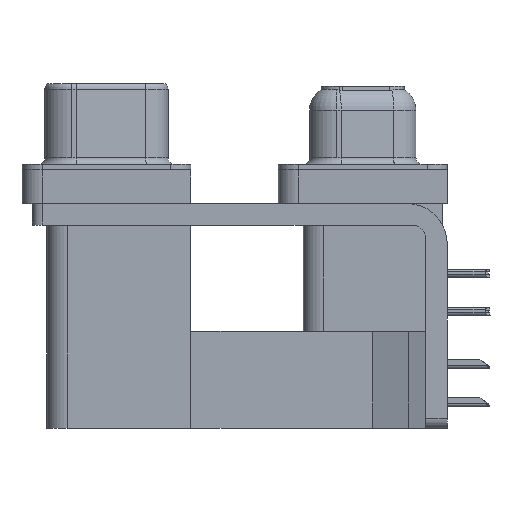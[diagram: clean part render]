
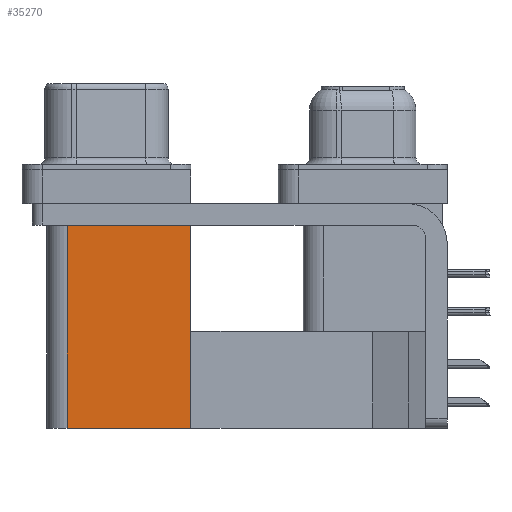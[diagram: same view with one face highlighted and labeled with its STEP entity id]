
A CAD part, left-side view. The second image highlights one B-rep face of the part: STEP entity #35270.
In plain terms, the highlighted planar face has unit normal (-1, 0, 0).
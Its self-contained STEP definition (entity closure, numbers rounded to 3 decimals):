
#54 = ORIENTED_EDGE ( 'NONE', *, *, #5511, .F. ) ;
#746 = FACE_OUTER_BOUND ( 'NONE', #6804, .T. ) ;
#1076 = VECTOR ( 'NONE', #1317, 1000. ) ;
#1317 = DIRECTION ( 'NONE',  ( 0., 1., 0. ) ) ;
#1485 = DIRECTION ( 'NONE',  ( 1., 0., 0. ) ) ;
#1719 = DIRECTION ( 'NONE',  ( 0., 0., 1. ) ) ;
#4281 = VERTEX_POINT ( 'NONE', #9733 ) ;
#5478 = LINE ( 'NONE', #19414, #6993 ) ;
#5511 = EDGE_CURVE ( 'NONE', #35885, #22457, #18679, .T. ) ;
#6804 = EDGE_LOOP ( 'NONE', ( #35954, #54, #20060, #24211 ) ) ;
#6993 = VECTOR ( 'NONE', #16777, 1000. ) ;
#9494 = EDGE_CURVE ( 'NONE', #33871, #35885, #5478, .T. ) ;
#9733 = CARTESIAN_POINT ( 'NONE',  ( 3.79, 12.775, -2.5 ) ) ;
#11912 = LINE ( 'NONE', #17920, #20626 ) ;
#12416 = CARTESIAN_POINT ( 'NONE',  ( 3.79, 21.975, -2.5 ) ) ;
#12964 = DIRECTION ( 'NONE',  ( 0., 0., -1. ) ) ;
#16777 = DIRECTION ( 'NONE',  ( 0., 1., 0. ) ) ;
#17920 = CARTESIAN_POINT ( 'NONE',  ( 3.79, 12.775, -19.2 ) ) ;
#18240 = EDGE_CURVE ( 'NONE', #33871, #4281, #11912, .T. ) ;
#18679 = LINE ( 'NONE', #33002, #27005 ) ;
#19414 = CARTESIAN_POINT ( 'NONE',  ( 3.79, 12.775, -19.2 ) ) ;
#20060 = ORIENTED_EDGE ( 'NONE', *, *, #9494, .F. ) ;
#20626 = VECTOR ( 'NONE', #32243, 1000. ) ;
#22457 = VERTEX_POINT ( 'NONE', #12416 ) ;
#24211 = ORIENTED_EDGE ( 'NONE', *, *, #18240, .T. ) ;
#27005 = VECTOR ( 'NONE', #1719, 1000. ) ;
#27107 = CARTESIAN_POINT ( 'NONE',  ( 3.79, 12.775, -19.2 ) ) ;
#28250 = AXIS2_PLACEMENT_3D ( 'NONE', #27107, #1485, #12964 ) ;
#28579 = CARTESIAN_POINT ( 'NONE',  ( 3.79, 12.775, -19.2 ) ) ;
#31033 = EDGE_CURVE ( 'NONE', #4281, #22457, #32777, .T. ) ;
#32216 = CARTESIAN_POINT ( 'NONE',  ( 3.79, 12.775, -2.5 ) ) ;
#32243 = DIRECTION ( 'NONE',  ( 0., 0., 1. ) ) ;
#32401 = PLANE ( 'NONE',  #28250 ) ;
#32777 = LINE ( 'NONE', #32216, #1076 ) ;
#33002 = CARTESIAN_POINT ( 'NONE',  ( 3.79, 21.975, -19.2 ) ) ;
#33871 = VERTEX_POINT ( 'NONE', #28579 ) ;
#35270 = ADVANCED_FACE ( 'NONE', ( #746 ), #32401, .F. ) ;
#35479 = CARTESIAN_POINT ( 'NONE',  ( 3.79, 21.975, -19.2 ) ) ;
#35885 = VERTEX_POINT ( 'NONE', #35479 ) ;
#35954 = ORIENTED_EDGE ( 'NONE', *, *, #31033, .T. ) ;
